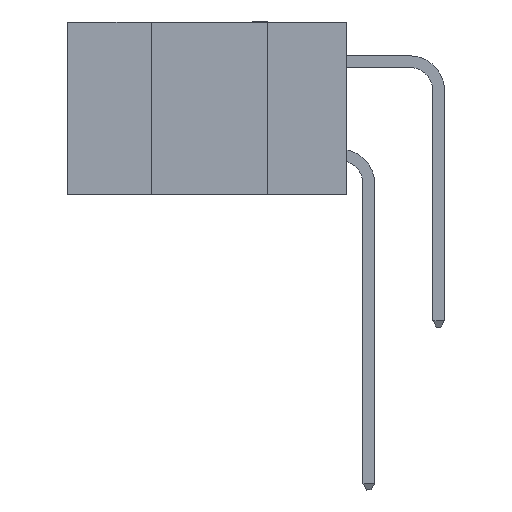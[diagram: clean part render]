
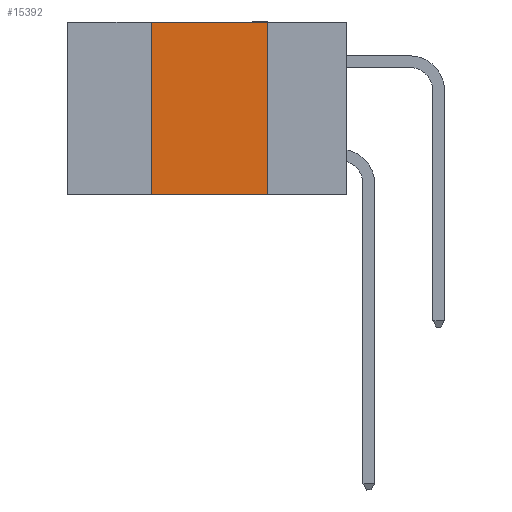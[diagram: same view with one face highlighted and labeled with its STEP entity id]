
A CAD part, left-side view. The second image highlights one B-rep face of the part: STEP entity #15392.
In plain terms, the highlighted planar face has unit normal (-1, 0, 0).
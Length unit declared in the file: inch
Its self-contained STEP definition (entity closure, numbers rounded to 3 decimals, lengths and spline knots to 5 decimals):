
#71 = CARTESIAN_POINT ( 'NONE',  ( 0., 0.17, 0. ) ) ;
#83 = VECTOR ( 'NONE', #21470, 39.37008 ) ;
#1356 = VERTEX_POINT ( 'NONE', #16614 ) ;
#1867 = VERTEX_POINT ( 'NONE', #4543 ) ;
#2255 = CARTESIAN_POINT ( 'NONE',  ( 0., 0.6, 0. ) ) ;
#2817 = CARTESIAN_POINT ( 'NONE',  ( 0., 0.17, 0. ) ) ;
#3010 = CARTESIAN_POINT ( 'NONE',  ( 0., 0.6, 0. ) ) ;
#4031 = ORIENTED_EDGE ( 'NONE', *, *, #14860, .T. ) ;
#4543 = CARTESIAN_POINT ( 'NONE',  ( 0., 0.42, 0. ) ) ;
#4776 = EDGE_CURVE ( 'NONE', #8280, #22894, #13143, .T. ) ;
#5496 = VECTOR ( 'NONE', #16674, 39.37008 ) ;
#6695 = LINE ( 'NONE', #19476, #83 ) ;
#6747 = VECTOR ( 'NONE', #12012, 39.37008 ) ;
#7222 = CARTESIAN_POINT ( 'NONE',  ( 0., 0.42, 0. ) ) ;
#8280 = VERTEX_POINT ( 'NONE', #2817 ) ;
#11293 = ORIENTED_EDGE ( 'NONE', *, *, #18892, .F. ) ;
#11898 = DIRECTION ( 'NONE',  ( 0., 0., -1. ) ) ;
#12012 = DIRECTION ( 'NONE',  ( 0., 0., -1. ) ) ;
#13143 = LINE ( 'NONE', #71, #6747 ) ;
#13725 = FACE_OUTER_BOUND ( 'NONE', #16233, .T. ) ;
#14860 = EDGE_CURVE ( 'NONE', #1356, #22894, #6695, .T. ) ;
#15392 = ADVANCED_FACE ( 'NONE', ( #13725 ), #18865, .F. ) ;
#16233 = EDGE_LOOP ( 'NONE', ( #17763, #11293, #17355, #4031 ) ) ;
#16614 = CARTESIAN_POINT ( 'NONE',  ( 0., 0.42, -0.37 ) ) ;
#16674 = DIRECTION ( 'NONE',  ( 0., -1., 0. ) ) ;
#17355 = ORIENTED_EDGE ( 'NONE', *, *, #19316, .F. ) ;
#17763 = ORIENTED_EDGE ( 'NONE', *, *, #4776, .F. ) ;
#18865 = PLANE ( 'NONE',  #22530 ) ;
#18869 = CARTESIAN_POINT ( 'NONE',  ( 0., 0.17, -0.37 ) ) ;
#18892 = EDGE_CURVE ( 'NONE', #1867, #8280, #20207, .T. ) ;
#19316 = EDGE_CURVE ( 'NONE', #1356, #1867, #21871, .T. ) ;
#19476 = CARTESIAN_POINT ( 'NONE',  ( 0., 0.6, -0.37 ) ) ;
#19607 = DIRECTION ( 'NONE',  ( 0., 0., 1. ) ) ;
#20207 = LINE ( 'NONE', #2255, #5496 ) ;
#21045 = VECTOR ( 'NONE', #19607, 39.37008 ) ;
#21470 = DIRECTION ( 'NONE',  ( 0., -1., 0. ) ) ;
#21871 = LINE ( 'NONE', #7222, #21045 ) ;
#22476 = DIRECTION ( 'NONE',  ( 1., 0., 0. ) ) ;
#22530 = AXIS2_PLACEMENT_3D ( 'NONE', #3010, #22476, #11898 ) ;
#22894 = VERTEX_POINT ( 'NONE', #18869 ) ;
